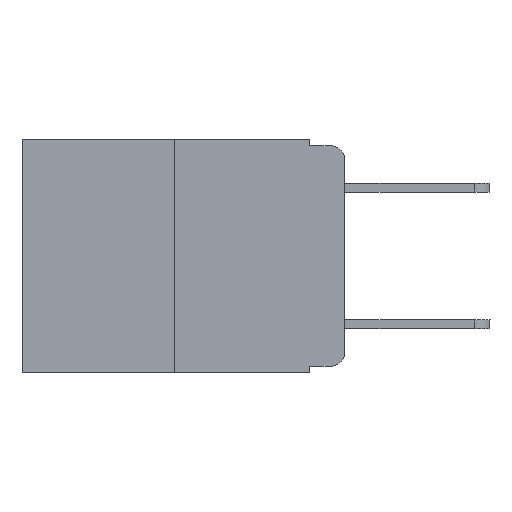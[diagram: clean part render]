
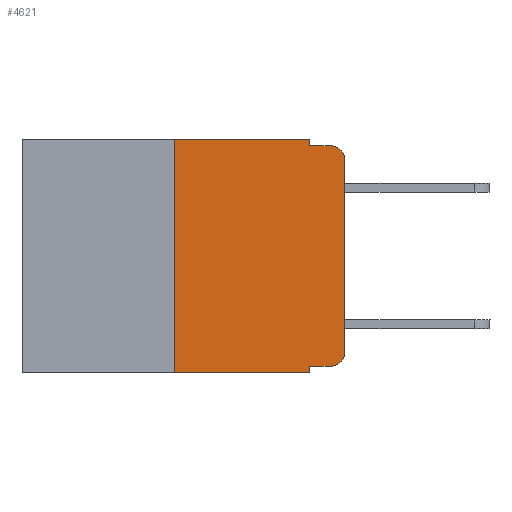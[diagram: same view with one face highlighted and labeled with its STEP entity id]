
A CAD part, left-side view. The second image highlights one B-rep face of the part: STEP entity #4621.
In plain terms, the highlighted planar face has unit normal (-1, 0, 0).
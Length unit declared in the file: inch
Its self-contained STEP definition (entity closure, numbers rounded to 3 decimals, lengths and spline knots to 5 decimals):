
#15 = CARTESIAN_POINT ( 'NONE',  ( 0., 0.473, 0. ) ) ;
#28 = CARTESIAN_POINT ( 'NONE',  ( 0., 0.473, -0.343 ) ) ;
#56 = CARTESIAN_POINT ( 'NONE',  ( 0., 0.02, -0.01 ) ) ;
#61 = VERTEX_POINT ( 'NONE', #7846 ) ;
#117 = ORIENTED_EDGE ( 'NONE', *, *, #9427, .T. ) ;
#606 = CIRCLE ( 'NONE', #7741, 0.02 ) ;
#782 = CARTESIAN_POINT ( 'NONE',  ( 0., 0.051, -0.01 ) ) ;
#912 = DIRECTION ( 'NONE',  ( 0., -1., 0. ) ) ;
#1064 = DIRECTION ( 'NONE',  ( 0., 0., -1. ) ) ;
#1184 = CARTESIAN_POINT ( 'NONE',  ( 0., 0.051, -0.343 ) ) ;
#1374 = VERTEX_POINT ( 'NONE', #4200 ) ;
#1590 = DIRECTION ( 'NONE',  ( 0., 0., -1. ) ) ;
#2181 = VECTOR ( 'NONE', #912, 39.37008 ) ;
#2309 = ORIENTED_EDGE ( 'NONE', *, *, #4530, .F. ) ;
#2538 = DIRECTION ( 'NONE',  ( -1., 0., 0. ) ) ;
#2784 = CARTESIAN_POINT ( 'NONE',  ( 0., 0.02, -0.03 ) ) ;
#2787 = VERTEX_POINT ( 'NONE', #4479 ) ;
#2836 = EDGE_CURVE ( 'NONE', #8976, #8958, #606, .T. ) ;
#3042 = VECTOR ( 'NONE', #4510, 39.37008 ) ;
#3211 = AXIS2_PLACEMENT_3D ( 'NONE', #8231, #2538, #1590 ) ;
#3277 = VERTEX_POINT ( 'NONE', #7072 ) ;
#3340 = CARTESIAN_POINT ( 'NONE',  ( 0., 0.473, 0. ) ) ;
#3355 = DIRECTION ( 'NONE',  ( 0., 0., -1. ) ) ;
#3589 = ORIENTED_EDGE ( 'NONE', *, *, #7709, .T. ) ;
#3627 = CARTESIAN_POINT ( 'NONE',  ( 0., 0.25, 0. ) ) ;
#3786 = VERTEX_POINT ( 'NONE', #7802 ) ;
#3787 = DIRECTION ( 'NONE',  ( 0., 0., 1. ) ) ;
#3920 = VERTEX_POINT ( 'NONE', #9710 ) ;
#4102 = VECTOR ( 'NONE', #3355, 39.37008 ) ;
#4185 = EDGE_CURVE ( 'NONE', #3786, #7352, #9006, .T. ) ;
#4200 = CARTESIAN_POINT ( 'NONE',  ( 0., 0.051, -0.01 ) ) ;
#4418 = CARTESIAN_POINT ( 'NONE',  ( 0., 0.051, 0. ) ) ;
#4432 = DIRECTION ( 'NONE',  ( -1., 0., 0. ) ) ;
#4479 = CARTESIAN_POINT ( 'NONE',  ( 0., 0., -0.313 ) ) ;
#4510 = DIRECTION ( 'NONE',  ( 0., 0., 1. ) ) ;
#4530 = EDGE_CURVE ( 'NONE', #61, #3786, #7224, .T. ) ;
#4617 = ORIENTED_EDGE ( 'NONE', *, *, #6074, .F. ) ;
#4621 = ADVANCED_FACE ( 'NONE', ( #10522 ), #7340, .F. ) ;
#4739 = VECTOR ( 'NONE', #3787, 39.37008 ) ;
#4835 = DIRECTION ( 'NONE',  ( 1., 0., 0. ) ) ;
#4941 = VECTOR ( 'NONE', #9801, 39.37008 ) ;
#4962 = CARTESIAN_POINT ( 'NONE',  ( 0., 0., -0.03 ) ) ;
#5236 = VECTOR ( 'NONE', #1064, 39.37008 ) ;
#5326 = ORIENTED_EDGE ( 'NONE', *, *, #4185, .F. ) ;
#5364 = ORIENTED_EDGE ( 'NONE', *, *, #7753, .F. ) ;
#5628 = DIRECTION ( 'NONE',  ( 0., -1., 0. ) ) ;
#5907 = EDGE_LOOP ( 'NONE', ( #9311, #9435, #7172, #4617, #5326, #2309, #9270, #5364, #3589, #117 ) ) ;
#6074 = EDGE_CURVE ( 'NONE', #7352, #1374, #9996, .T. ) ;
#6499 = LINE ( 'NONE', #8932, #2181 ) ;
#6581 = LINE ( 'NONE', #782, #10010 ) ;
#7072 = CARTESIAN_POINT ( 'NONE',  ( 0., 0.051, -0.333 ) ) ;
#7172 = ORIENTED_EDGE ( 'NONE', *, *, #9395, .F. ) ;
#7224 = LINE ( 'NONE', #3627, #4739 ) ;
#7323 = LINE ( 'NONE', #28, #4941 ) ;
#7340 = PLANE ( 'NONE',  #9664 ) ;
#7352 = VERTEX_POINT ( 'NONE', #7614 ) ;
#7555 = CARTESIAN_POINT ( 'NONE',  ( 0., 0.051, 0. ) ) ;
#7614 = CARTESIAN_POINT ( 'NONE',  ( 0., 0.051, 0. ) ) ;
#7678 = DIRECTION ( 'NONE',  ( 0., 0., -1. ) ) ;
#7709 = EDGE_CURVE ( 'NONE', #3277, #3920, #6499, .T. ) ;
#7741 = AXIS2_PLACEMENT_3D ( 'NONE', #2784, #4432, #7678 ) ;
#7753 = EDGE_CURVE ( 'NONE', #3277, #8610, #8355, .T. ) ;
#7799 = CIRCLE ( 'NONE', #3211, 0.02 ) ;
#7802 = CARTESIAN_POINT ( 'NONE',  ( 0., 0.25, 0. ) ) ;
#7846 = CARTESIAN_POINT ( 'NONE',  ( 0., 0.25, -0.343 ) ) ;
#8214 = DIRECTION ( 'NONE',  ( 0., -1., 0. ) ) ;
#8231 = CARTESIAN_POINT ( 'NONE',  ( 0., 0.02, -0.313 ) ) ;
#8355 = LINE ( 'NONE', #7555, #5236 ) ;
#8455 = CARTESIAN_POINT ( 'NONE',  ( 0., 0., 0. ) ) ;
#8610 = VERTEX_POINT ( 'NONE', #1184 ) ;
#8932 = CARTESIAN_POINT ( 'NONE',  ( 0., 0.051, -0.333 ) ) ;
#8958 = VERTEX_POINT ( 'NONE', #56 ) ;
#8976 = VERTEX_POINT ( 'NONE', #4962 ) ;
#9006 = LINE ( 'NONE', #15, #10132 ) ;
#9030 = DIRECTION ( 'NONE',  ( 0., 0., -1. ) ) ;
#9034 = EDGE_CURVE ( 'NONE', #2787, #8976, #10145, .T. ) ;
#9270 = ORIENTED_EDGE ( 'NONE', *, *, #9785, .T. ) ;
#9311 = ORIENTED_EDGE ( 'NONE', *, *, #9034, .T. ) ;
#9395 = EDGE_CURVE ( 'NONE', #1374, #8958, #6581, .T. ) ;
#9427 = EDGE_CURVE ( 'NONE', #3920, #2787, #7799, .T. ) ;
#9435 = ORIENTED_EDGE ( 'NONE', *, *, #2836, .T. ) ;
#9664 = AXIS2_PLACEMENT_3D ( 'NONE', #3340, #4835, #9030 ) ;
#9710 = CARTESIAN_POINT ( 'NONE',  ( 0., 0.02, -0.333 ) ) ;
#9785 = EDGE_CURVE ( 'NONE', #61, #8610, #7323, .T. ) ;
#9801 = DIRECTION ( 'NONE',  ( 0., -1., 0. ) ) ;
#9996 = LINE ( 'NONE', #4418, #4102 ) ;
#10010 = VECTOR ( 'NONE', #5628, 39.37008 ) ;
#10132 = VECTOR ( 'NONE', #8214, 39.37008 ) ;
#10145 = LINE ( 'NONE', #8455, #3042 ) ;
#10522 = FACE_OUTER_BOUND ( 'NONE', #5907, .T. ) ;
